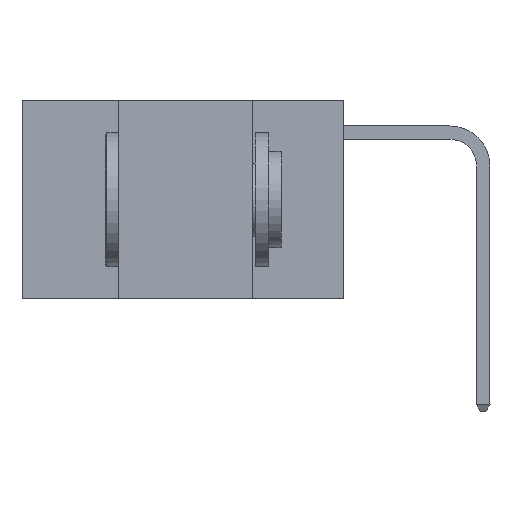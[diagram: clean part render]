
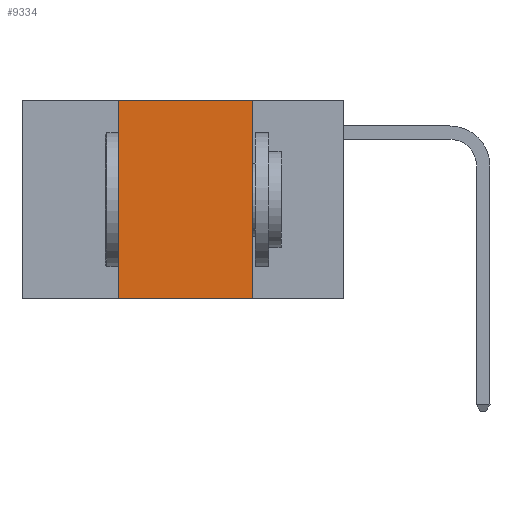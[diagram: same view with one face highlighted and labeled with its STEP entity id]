
A CAD part, left-side view. The second image highlights one B-rep face of the part: STEP entity #9334.
In plain terms, the highlighted planar face has unit normal (-1, 0, 0).
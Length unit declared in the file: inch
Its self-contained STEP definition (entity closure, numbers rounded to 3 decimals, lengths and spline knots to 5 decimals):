
#370 = CARTESIAN_POINT ( 'NONE',  ( 0., 0.6, -0.37 ) ) ;
#552 = EDGE_CURVE ( 'NONE', #7119, #6239, #1567, .T. ) ;
#673 = DIRECTION ( 'NONE',  ( 0., -1., 0. ) ) ;
#885 = CARTESIAN_POINT ( 'NONE',  ( 0., 0.6, 0. ) ) ;
#1339 = LINE ( 'NONE', #10753, #11818 ) ;
#1567 = LINE ( 'NONE', #885, #6766 ) ;
#2325 = VECTOR ( 'NONE', #13051, 39.37008 ) ;
#2417 = VECTOR ( 'NONE', #12605, 39.37008 ) ;
#2514 = ORIENTED_EDGE ( 'NONE', *, *, #2620, .F. ) ;
#2620 = EDGE_CURVE ( 'NONE', #3928, #7119, #1339, .T. ) ;
#2823 = PLANE ( 'NONE',  #12317 ) ;
#3169 = ORIENTED_EDGE ( 'NONE', *, *, #8092, .F. ) ;
#3299 = CARTESIAN_POINT ( 'NONE',  ( 0., 0.17, -0.37 ) ) ;
#3909 = DIRECTION ( 'NONE',  ( 0., 0., -1. ) ) ;
#3928 = VERTEX_POINT ( 'NONE', #7499 ) ;
#4208 = ORIENTED_EDGE ( 'NONE', *, *, #552, .F. ) ;
#5151 = LINE ( 'NONE', #370, #2417 ) ;
#5402 = ORIENTED_EDGE ( 'NONE', *, *, #10421, .T. ) ;
#5945 = CARTESIAN_POINT ( 'NONE',  ( 0., 0.17, 0. ) ) ;
#6136 = CARTESIAN_POINT ( 'NONE',  ( 0., 0.17, 0. ) ) ;
#6239 = VERTEX_POINT ( 'NONE', #5945 ) ;
#6563 = CARTESIAN_POINT ( 'NONE',  ( 0., 0.42, 0. ) ) ;
#6766 = VECTOR ( 'NONE', #673, 39.37008 ) ;
#7119 = VERTEX_POINT ( 'NONE', #6563 ) ;
#7459 = LINE ( 'NONE', #6136, #2325 ) ;
#7499 = CARTESIAN_POINT ( 'NONE',  ( 0., 0.42, -0.37 ) ) ;
#8092 = EDGE_CURVE ( 'NONE', #6239, #11438, #7459, .T. ) ;
#8771 = DIRECTION ( 'NONE',  ( 0., 0., 1. ) ) ;
#8887 = CARTESIAN_POINT ( 'NONE',  ( 0., 0.6, 0. ) ) ;
#9334 = ADVANCED_FACE ( 'NONE', ( #12674 ), #2823, .F. ) ;
#9909 = EDGE_LOOP ( 'NONE', ( #3169, #4208, #2514, #5402 ) ) ;
#9920 = DIRECTION ( 'NONE',  ( 1., 0., 0. ) ) ;
#10421 = EDGE_CURVE ( 'NONE', #3928, #11438, #5151, .T. ) ;
#10753 = CARTESIAN_POINT ( 'NONE',  ( 0., 0.42, 0. ) ) ;
#11438 = VERTEX_POINT ( 'NONE', #3299 ) ;
#11818 = VECTOR ( 'NONE', #8771, 39.37008 ) ;
#12317 = AXIS2_PLACEMENT_3D ( 'NONE', #8887, #9920, #3909 ) ;
#12605 = DIRECTION ( 'NONE',  ( 0., -1., 0. ) ) ;
#12674 = FACE_OUTER_BOUND ( 'NONE', #9909, .T. ) ;
#13051 = DIRECTION ( 'NONE',  ( 0., 0., -1. ) ) ;
